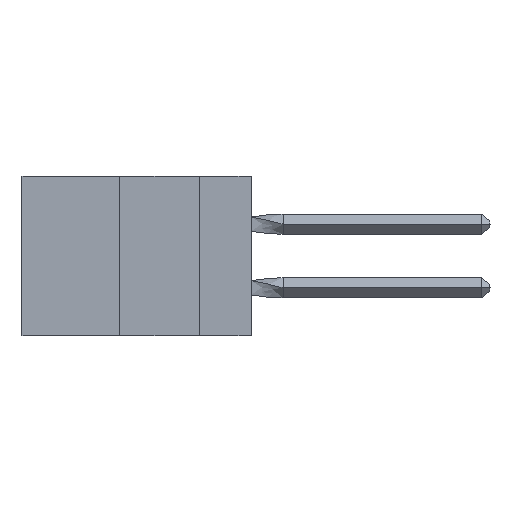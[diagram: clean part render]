
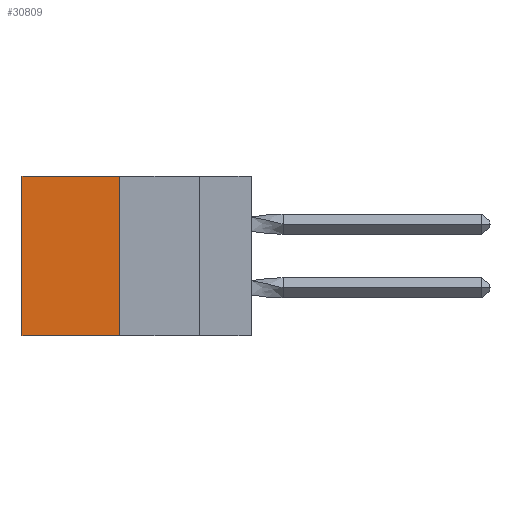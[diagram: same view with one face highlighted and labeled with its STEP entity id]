
A CAD part, left-side view. The second image highlights one B-rep face of the part: STEP entity #30809.
In plain terms, the highlighted planar face has unit normal (-1, 0, 0).
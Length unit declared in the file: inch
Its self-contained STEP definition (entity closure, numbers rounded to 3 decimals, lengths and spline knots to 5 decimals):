
#494 = EDGE_CURVE ( 'NONE', #21724, #17664, #13567, .T. ) ;
#1277 = LINE ( 'NONE', #5345, #30075 ) ;
#1410 = VERTEX_POINT ( 'NONE', #15361 ) ;
#1515 = DIRECTION ( 'NONE',  ( 0., 1., 0. ) ) ;
#3486 = CARTESIAN_POINT ( 'NONE',  ( 0.305, 0.413, 0. ) ) ;
#4257 = EDGE_CURVE ( 'NONE', #18896, #21724, #34720, .T. ) ;
#4336 = ORIENTED_EDGE ( 'NONE', *, *, #494, .F. ) ;
#4375 = DIRECTION ( 'NONE',  ( 0., 0., -1. ) ) ;
#5345 = CARTESIAN_POINT ( 'NONE',  ( 0.305, 0.413, 0. ) ) ;
#6644 = EDGE_CURVE ( 'NONE', #1410, #17664, #13916, .T. ) ;
#8223 = CARTESIAN_POINT ( 'NONE',  ( 0.305, 0.413, -0.5 ) ) ;
#9939 = VECTOR ( 'NONE', #22007, 39.37008 ) ;
#13349 = EDGE_CURVE ( 'NONE', #18896, #1410, #1277, .T. ) ;
#13567 = LINE ( 'NONE', #8223, #26442 ) ;
#13916 = LINE ( 'NONE', #33817, #21847 ) ;
#14799 = DIRECTION ( 'NONE',  ( 0., 1., 0. ) ) ;
#15361 = CARTESIAN_POINT ( 'NONE',  ( 0.305, 0.72, 0. ) ) ;
#17664 = VERTEX_POINT ( 'NONE', #37839 ) ;
#18896 = VERTEX_POINT ( 'NONE', #3486 ) ;
#19108 = CARTESIAN_POINT ( 'NONE',  ( 0.305, 0.413, -0.5 ) ) ;
#19655 = PLANE ( 'NONE',  #35795 ) ;
#21724 = VERTEX_POINT ( 'NONE', #36291 ) ;
#21847 = VECTOR ( 'NONE', #27609, 39.37008 ) ;
#22007 = DIRECTION ( 'NONE',  ( 0., 0., -1. ) ) ;
#22946 = DIRECTION ( 'NONE',  ( 1., 0., 0. ) ) ;
#24903 = CARTESIAN_POINT ( 'NONE',  ( 0.305, 0.413, -0.5 ) ) ;
#26442 = VECTOR ( 'NONE', #1515, 39.37008 ) ;
#27609 = DIRECTION ( 'NONE',  ( 0., 0., -1. ) ) ;
#27945 = ORIENTED_EDGE ( 'NONE', *, *, #4257, .F. ) ;
#30075 = VECTOR ( 'NONE', #14799, 39.37008 ) ;
#30809 = ADVANCED_FACE ( 'NONE', ( #31474 ), #19655, .F. ) ;
#31474 = FACE_OUTER_BOUND ( 'NONE', #35393, .T. ) ;
#33817 = CARTESIAN_POINT ( 'NONE',  ( 0.305, 0.72, -0.5 ) ) ;
#34720 = LINE ( 'NONE', #24903, #9939 ) ;
#35393 = EDGE_LOOP ( 'NONE', ( #39528, #4336, #27945, #40549 ) ) ;
#35795 = AXIS2_PLACEMENT_3D ( 'NONE', #19108, #22946, #4375 ) ;
#36291 = CARTESIAN_POINT ( 'NONE',  ( 0.305, 0.413, -0.5 ) ) ;
#37839 = CARTESIAN_POINT ( 'NONE',  ( 0.305, 0.72, -0.5 ) ) ;
#39528 = ORIENTED_EDGE ( 'NONE', *, *, #6644, .T. ) ;
#40549 = ORIENTED_EDGE ( 'NONE', *, *, #13349, .T. ) ;
